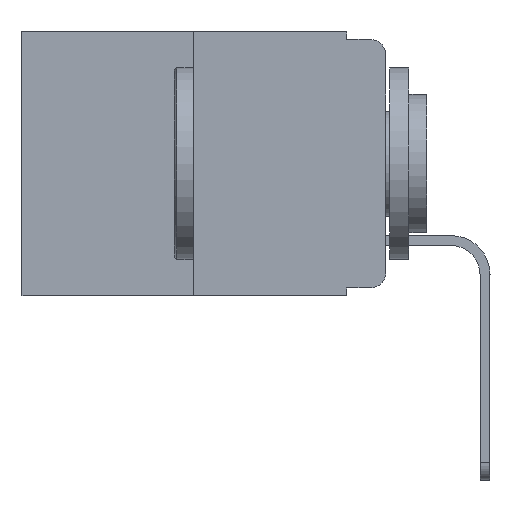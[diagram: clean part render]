
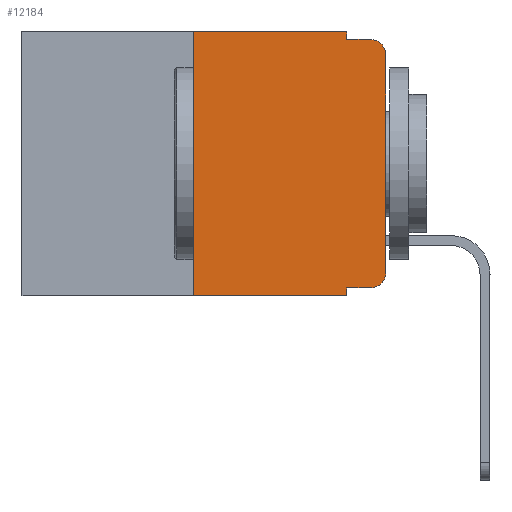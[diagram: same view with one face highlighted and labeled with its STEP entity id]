
A CAD part, left-side view. The second image highlights one B-rep face of the part: STEP entity #12184.
In plain terms, the highlighted planar face has unit normal (-1, 0, 0).
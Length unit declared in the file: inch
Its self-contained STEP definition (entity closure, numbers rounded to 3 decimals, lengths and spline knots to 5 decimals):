
#607 = LINE ( 'NONE', #16194, #19904 ) ;
#804 = VERTEX_POINT ( 'NONE', #14787 ) ;
#911 = DIRECTION ( 'NONE',  ( 0., 0., -1. ) ) ;
#1182 = DIRECTION ( 'NONE',  ( 0., -1., 0. ) ) ;
#1323 = EDGE_CURVE ( 'NONE', #10665, #13269, #607, .T. ) ;
#1370 = VERTEX_POINT ( 'NONE', #19954 ) ;
#1378 = ORIENTED_EDGE ( 'NONE', *, *, #10255, .T. ) ;
#1634 = EDGE_CURVE ( 'NONE', #19611, #7855, #12522, .T. ) ;
#1849 = LINE ( 'NONE', #7629, #3109 ) ;
#2526 = PLANE ( 'NONE',  #12955 ) ;
#2871 = EDGE_CURVE ( 'NONE', #4362, #6473, #4895, .T. ) ;
#3109 = VECTOR ( 'NONE', #10528, 39.37008 ) ;
#3868 = DIRECTION ( 'NONE',  ( 0., 0., 1. ) ) ;
#3872 = CARTESIAN_POINT ( 'NONE',  ( 0., 0.051, 0. ) ) ;
#4035 = CIRCLE ( 'NONE', #5481, 0.02 ) ;
#4196 = VECTOR ( 'NONE', #3868, 39.37008 ) ;
#4362 = VERTEX_POINT ( 'NONE', #10082 ) ;
#4445 = ORIENTED_EDGE ( 'NONE', *, *, #19216, .F. ) ;
#4530 = FACE_OUTER_BOUND ( 'NONE', #4792, .T. ) ;
#4550 = CARTESIAN_POINT ( 'NONE',  ( 0., 0.051, 0. ) ) ;
#4792 = EDGE_LOOP ( 'NONE', ( #18428, #10405, #17138, #9426, #4445, #10566, #6726, #6313, #1378, #5611 ) ) ;
#4895 = LINE ( 'NONE', #18952, #13005 ) ;
#5481 = AXIS2_PLACEMENT_3D ( 'NONE', #17328, #18965, #20676 ) ;
#5611 = ORIENTED_EDGE ( 'NONE', *, *, #18790, .T. ) ;
#5817 = CARTESIAN_POINT ( 'NONE',  ( 0., 0.02, -0.01 ) ) ;
#6175 = VECTOR ( 'NONE', #6448, 39.37008 ) ;
#6286 = DIRECTION ( 'NONE',  ( 0., -1., 0. ) ) ;
#6313 = ORIENTED_EDGE ( 'NONE', *, *, #20842, .F. ) ;
#6448 = DIRECTION ( 'NONE',  ( 0., 0., -1. ) ) ;
#6473 = VERTEX_POINT ( 'NONE', #5817 ) ;
#6726 = ORIENTED_EDGE ( 'NONE', *, *, #12270, .T. ) ;
#7629 = CARTESIAN_POINT ( 'NONE',  ( 0., 0.051, -0.333 ) ) ;
#7855 = VERTEX_POINT ( 'NONE', #8245 ) ;
#8245 = CARTESIAN_POINT ( 'NONE',  ( 0., 0., -0.03 ) ) ;
#8840 = LINE ( 'NONE', #3872, #17990 ) ;
#8967 = DIRECTION ( 'NONE',  ( 1., 0., 0. ) ) ;
#9016 = DIRECTION ( 'NONE',  ( 0., -1., 0. ) ) ;
#9426 = ORIENTED_EDGE ( 'NONE', *, *, #15512, .F. ) ;
#9573 = CIRCLE ( 'NONE', #14052, 0.02 ) ;
#10082 = CARTESIAN_POINT ( 'NONE',  ( 0., 0.051, -0.01 ) ) ;
#10182 = CARTESIAN_POINT ( 'NONE',  ( 0., 0.02, -0.333 ) ) ;
#10255 = EDGE_CURVE ( 'NONE', #804, #14067, #1849, .T. ) ;
#10405 = ORIENTED_EDGE ( 'NONE', *, *, #12293, .T. ) ;
#10528 = DIRECTION ( 'NONE',  ( 0., -1., 0. ) ) ;
#10566 = ORIENTED_EDGE ( 'NONE', *, *, #1323, .F. ) ;
#10665 = VERTEX_POINT ( 'NONE', #13494 ) ;
#11084 = CARTESIAN_POINT ( 'NONE',  ( 0., 0.473, -0.343 ) ) ;
#12184 = ADVANCED_FACE ( 'NONE', ( #4530 ), #2526, .F. ) ;
#12270 = EDGE_CURVE ( 'NONE', #10665, #1370, #15426, .T. ) ;
#12293 = EDGE_CURVE ( 'NONE', #7855, #6473, #9573, .T. ) ;
#12522 = LINE ( 'NONE', #18121, #4196 ) ;
#12588 = DIRECTION ( 'NONE',  ( 0., 0., -1. ) ) ;
#12731 = LINE ( 'NONE', #16014, #18824 ) ;
#12955 = AXIS2_PLACEMENT_3D ( 'NONE', #14083, #8967, #911 ) ;
#13005 = VECTOR ( 'NONE', #9016, 39.37008 ) ;
#13269 = VERTEX_POINT ( 'NONE', #15305 ) ;
#13415 = DIRECTION ( 'NONE',  ( 0., 0., 1. ) ) ;
#13494 = CARTESIAN_POINT ( 'NONE',  ( 0., 0.25, -0.343 ) ) ;
#13874 = CARTESIAN_POINT ( 'NONE',  ( 0., 0., -0.313 ) ) ;
#14052 = AXIS2_PLACEMENT_3D ( 'NONE', #19193, #17485, #12588 ) ;
#14067 = VERTEX_POINT ( 'NONE', #10182 ) ;
#14083 = CARTESIAN_POINT ( 'NONE',  ( 0., 0.473, 0. ) ) ;
#14787 = CARTESIAN_POINT ( 'NONE',  ( 0., 0.051, -0.333 ) ) ;
#14879 = CARTESIAN_POINT ( 'NONE',  ( 0., 0.051, 0. ) ) ;
#15305 = CARTESIAN_POINT ( 'NONE',  ( 0., 0.25, 0. ) ) ;
#15426 = LINE ( 'NONE', #11084, #18726 ) ;
#15512 = EDGE_CURVE ( 'NONE', #17556, #4362, #19881, .T. ) ;
#16014 = CARTESIAN_POINT ( 'NONE',  ( 0., 0.473, 0. ) ) ;
#16194 = CARTESIAN_POINT ( 'NONE',  ( 0., 0.25, 0. ) ) ;
#16699 = DIRECTION ( 'NONE',  ( 0., 0., -1. ) ) ;
#17138 = ORIENTED_EDGE ( 'NONE', *, *, #2871, .F. ) ;
#17328 = CARTESIAN_POINT ( 'NONE',  ( 0., 0.02, -0.313 ) ) ;
#17485 = DIRECTION ( 'NONE',  ( -1., 0., 0. ) ) ;
#17556 = VERTEX_POINT ( 'NONE', #14879 ) ;
#17990 = VECTOR ( 'NONE', #16699, 39.37008 ) ;
#18121 = CARTESIAN_POINT ( 'NONE',  ( 0., 0., 0. ) ) ;
#18428 = ORIENTED_EDGE ( 'NONE', *, *, #1634, .T. ) ;
#18726 = VECTOR ( 'NONE', #1182, 39.37008 ) ;
#18790 = EDGE_CURVE ( 'NONE', #14067, #19611, #4035, .T. ) ;
#18824 = VECTOR ( 'NONE', #6286, 39.37008 ) ;
#18952 = CARTESIAN_POINT ( 'NONE',  ( 0., 0.051, -0.01 ) ) ;
#18965 = DIRECTION ( 'NONE',  ( -1., 0., 0. ) ) ;
#19193 = CARTESIAN_POINT ( 'NONE',  ( 0., 0.02, -0.03 ) ) ;
#19216 = EDGE_CURVE ( 'NONE', #13269, #17556, #12731, .T. ) ;
#19611 = VERTEX_POINT ( 'NONE', #13874 ) ;
#19881 = LINE ( 'NONE', #4550, #6175 ) ;
#19904 = VECTOR ( 'NONE', #13415, 39.37008 ) ;
#19954 = CARTESIAN_POINT ( 'NONE',  ( 0., 0.051, -0.343 ) ) ;
#20676 = DIRECTION ( 'NONE',  ( 0., 0., -1. ) ) ;
#20842 = EDGE_CURVE ( 'NONE', #804, #1370, #8840, .T. ) ;
